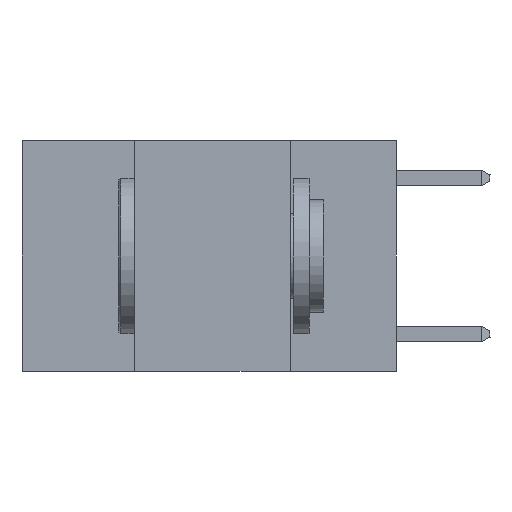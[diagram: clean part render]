
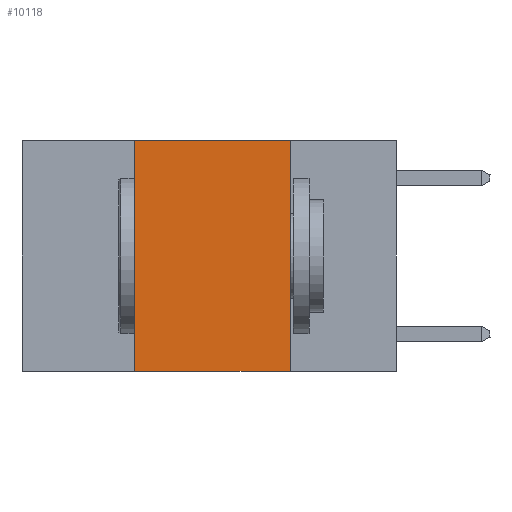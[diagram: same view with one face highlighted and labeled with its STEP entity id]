
A CAD part, left-side view. The second image highlights one B-rep face of the part: STEP entity #10118.
In plain terms, the highlighted planar face has unit normal (-1, 0, 0).
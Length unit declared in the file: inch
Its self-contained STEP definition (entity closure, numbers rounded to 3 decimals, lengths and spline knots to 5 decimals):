
#175 = VERTEX_POINT ( 'NONE', #6641 ) ;
#374 = CARTESIAN_POINT ( 'NONE',  ( 0., 0.42, 0. ) ) ;
#834 = VECTOR ( 'NONE', #12663, 39.37008 ) ;
#1138 = DIRECTION ( 'NONE',  ( 0., 0., 1. ) ) ;
#1321 = CARTESIAN_POINT ( 'NONE',  ( 0., 0.6, 0. ) ) ;
#1487 = LINE ( 'NONE', #6613, #16223 ) ;
#1566 = VERTEX_POINT ( 'NONE', #7340 ) ;
#1605 = VECTOR ( 'NONE', #9910, 39.37008 ) ;
#2111 = EDGE_CURVE ( 'NONE', #175, #1566, #12318, .T. ) ;
#2576 = EDGE_CURVE ( 'NONE', #9928, #4678, #5242, .T. ) ;
#3555 = CARTESIAN_POINT ( 'NONE',  ( 0., 0.17, 0. ) ) ;
#4032 = ORIENTED_EDGE ( 'NONE', *, *, #4763, .F. ) ;
#4470 = EDGE_CURVE ( 'NONE', #9928, #1566, #14822, .T. ) ;
#4678 = VERTEX_POINT ( 'NONE', #374 ) ;
#4763 = EDGE_CURVE ( 'NONE', #4678, #175, #1487, .T. ) ;
#4934 = PLANE ( 'NONE',  #13536 ) ;
#5242 = LINE ( 'NONE', #7574, #5937 ) ;
#5636 = CARTESIAN_POINT ( 'NONE',  ( 0., 0.42, -0.37 ) ) ;
#5937 = VECTOR ( 'NONE', #1138, 39.37008 ) ;
#6202 = FACE_OUTER_BOUND ( 'NONE', #12977, .T. ) ;
#6365 = DIRECTION ( 'NONE',  ( 0., 0., -1. ) ) ;
#6613 = CARTESIAN_POINT ( 'NONE',  ( 0., 0.6, 0. ) ) ;
#6641 = CARTESIAN_POINT ( 'NONE',  ( 0., 0.17, 0. ) ) ;
#7340 = CARTESIAN_POINT ( 'NONE',  ( 0., 0.17, -0.37 ) ) ;
#7574 = CARTESIAN_POINT ( 'NONE',  ( 0., 0.42, 0. ) ) ;
#7682 = CARTESIAN_POINT ( 'NONE',  ( 0., 0.6, -0.37 ) ) ;
#8304 = ORIENTED_EDGE ( 'NONE', *, *, #2576, .F. ) ;
#8784 = ORIENTED_EDGE ( 'NONE', *, *, #4470, .T. ) ;
#9910 = DIRECTION ( 'NONE',  ( 0., -1., 0. ) ) ;
#9928 = VERTEX_POINT ( 'NONE', #5636 ) ;
#10118 = ADVANCED_FACE ( 'NONE', ( #6202 ), #4934, .F. ) ;
#12318 = LINE ( 'NONE', #3555, #834 ) ;
#12663 = DIRECTION ( 'NONE',  ( 0., 0., -1. ) ) ;
#12815 = DIRECTION ( 'NONE',  ( 1., 0., 0. ) ) ;
#12977 = EDGE_LOOP ( 'NONE', ( #15286, #4032, #8304, #8784 ) ) ;
#13536 = AXIS2_PLACEMENT_3D ( 'NONE', #1321, #12815, #6365 ) ;
#14822 = LINE ( 'NONE', #7682, #1605 ) ;
#15286 = ORIENTED_EDGE ( 'NONE', *, *, #2111, .F. ) ;
#16223 = VECTOR ( 'NONE', #16403, 39.37008 ) ;
#16403 = DIRECTION ( 'NONE',  ( 0., -1., 0. ) ) ;
